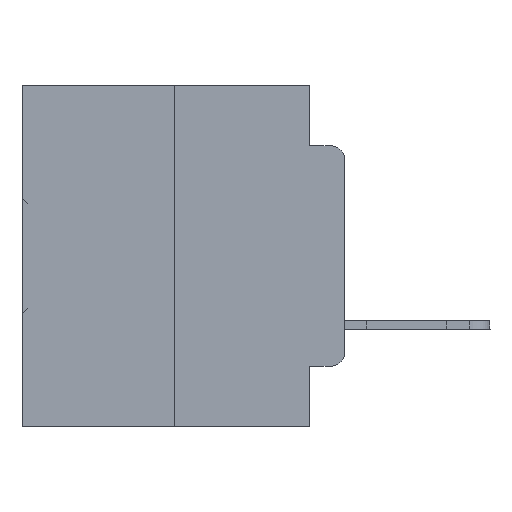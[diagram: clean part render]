
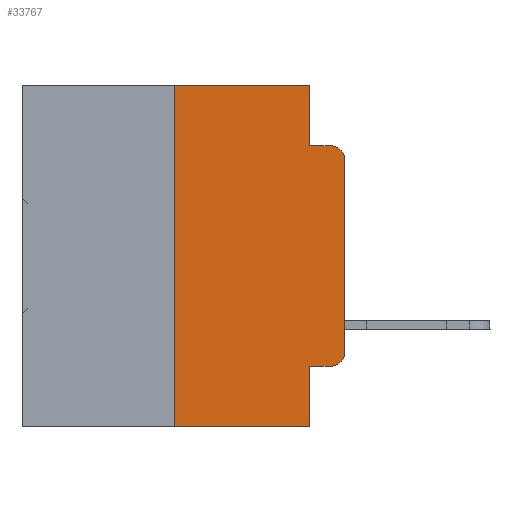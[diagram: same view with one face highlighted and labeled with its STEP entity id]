
A CAD part, left-side view. The second image highlights one B-rep face of the part: STEP entity #33767.
In plain terms, the highlighted planar face has unit normal (-1, 0, 0).
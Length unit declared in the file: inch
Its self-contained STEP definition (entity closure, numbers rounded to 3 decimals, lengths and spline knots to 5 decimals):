
#366 = DIRECTION ( 'NONE',  ( 0., 0., 1. ) ) ;
#1430 = VERTEX_POINT ( 'NONE', #19132 ) ;
#1471 = CARTESIAN_POINT ( 'NONE',  ( 0., 0.051, -0.4115 ) ) ;
#1493 = AXIS2_PLACEMENT_3D ( 'NONE', #34235, #16248, #6735 ) ;
#1638 = EDGE_CURVE ( 'NONE', #22404, #16948, #2850, .T. ) ;
#1696 = LINE ( 'NONE', #15486, #4446 ) ;
#2161 = DIRECTION ( 'NONE',  ( 0., -1., 0. ) ) ;
#2497 = LINE ( 'NONE', #13567, #11631 ) ;
#2709 = CARTESIAN_POINT ( 'NONE',  ( 0., 0.051, 0. ) ) ;
#2835 = ORIENTED_EDGE ( 'NONE', *, *, #12323, .F. ) ;
#2850 = CIRCLE ( 'NONE', #23720, 0.02 ) ;
#3597 = EDGE_CURVE ( 'NONE', #16376, #22404, #8184, .T. ) ;
#3764 = DIRECTION ( 'NONE',  ( 0., 0., 1. ) ) ;
#3869 = EDGE_CURVE ( 'NONE', #33502, #10345, #29828, .T. ) ;
#4326 = VERTEX_POINT ( 'NONE', #13324 ) ;
#4446 = VECTOR ( 'NONE', #26529, 39.37008 ) ;
#4755 = EDGE_CURVE ( 'NONE', #4326, #1430, #1696, .T. ) ;
#5610 = EDGE_CURVE ( 'NONE', #16376, #1430, #15595, .T. ) ;
#5778 = PLANE ( 'NONE',  #19825 ) ;
#5796 = ORIENTED_EDGE ( 'NONE', *, *, #15670, .F. ) ;
#6735 = DIRECTION ( 'NONE',  ( 0., 0., -1. ) ) ;
#7134 = EDGE_LOOP ( 'NONE', ( #18566, #29889, #5796, #25810, #19555, #2835, #34862, #23384, #22696, #13065 ) ) ;
#8184 = LINE ( 'NONE', #18720, #30967 ) ;
#10300 = LINE ( 'NONE', #13361, #29203 ) ;
#10345 = VERTEX_POINT ( 'NONE', #12587 ) ;
#10522 = DIRECTION ( 'NONE',  ( 1., 0., 0. ) ) ;
#11631 = VECTOR ( 'NONE', #2161, 39.37008 ) ;
#12323 = EDGE_CURVE ( 'NONE', #4326, #27994, #22105, .T. ) ;
#12352 = CARTESIAN_POINT ( 'NONE',  ( 0., 0.051, 0. ) ) ;
#12587 = CARTESIAN_POINT ( 'NONE',  ( 0., 0.02, -0.0885 ) ) ;
#13065 = ORIENTED_EDGE ( 'NONE', *, *, #1638, .T. ) ;
#13207 = CARTESIAN_POINT ( 'NONE',  ( 0., 0., -0.3915 ) ) ;
#13252 = CARTESIAN_POINT ( 'NONE',  ( 0., 0.473, 0. ) ) ;
#13324 = CARTESIAN_POINT ( 'NONE',  ( 0., 0.25, -0.5 ) ) ;
#13361 = CARTESIAN_POINT ( 'NONE',  ( 0., 0.051, -0.0885 ) ) ;
#13567 = CARTESIAN_POINT ( 'NONE',  ( 0., 0.473, 0. ) ) ;
#14799 = DIRECTION ( 'NONE',  ( 0., 0., -1. ) ) ;
#15486 = CARTESIAN_POINT ( 'NONE',  ( 0., 0.473, -0.5 ) ) ;
#15595 = LINE ( 'NONE', #26110, #34476 ) ;
#15670 = EDGE_CURVE ( 'NONE', #16125, #10345, #10300, .T. ) ;
#16125 = VERTEX_POINT ( 'NONE', #19430 ) ;
#16248 = DIRECTION ( 'NONE',  ( -1., 0., 0. ) ) ;
#16376 = VERTEX_POINT ( 'NONE', #1471 ) ;
#16539 = VERTEX_POINT ( 'NONE', #2709 ) ;
#16942 = VECTOR ( 'NONE', #17798, 39.37008 ) ;
#16948 = VERTEX_POINT ( 'NONE', #13207 ) ;
#17008 = CARTESIAN_POINT ( 'NONE',  ( 0., 0.02, -0.4115 ) ) ;
#17691 = CARTESIAN_POINT ( 'NONE',  ( 0., 0.02, -0.3915 ) ) ;
#17798 = DIRECTION ( 'NONE',  ( 0., 0., -1. ) ) ;
#18486 = DIRECTION ( 'NONE',  ( 0., 0., -1. ) ) ;
#18566 = ORIENTED_EDGE ( 'NONE', *, *, #35707, .T. ) ;
#18720 = CARTESIAN_POINT ( 'NONE',  ( 0., 0.051, -0.4115 ) ) ;
#19132 = CARTESIAN_POINT ( 'NONE',  ( 0., 0.051, -0.5 ) ) ;
#19430 = CARTESIAN_POINT ( 'NONE',  ( 0., 0.051, -0.0885 ) ) ;
#19555 = ORIENTED_EDGE ( 'NONE', *, *, #31768, .F. ) ;
#19825 = AXIS2_PLACEMENT_3D ( 'NONE', #13252, #10522, #27018 ) ;
#19963 = VECTOR ( 'NONE', #3764, 39.37008 ) ;
#20497 = LINE ( 'NONE', #12352, #16942 ) ;
#22105 = LINE ( 'NONE', #27718, #27798 ) ;
#22404 = VERTEX_POINT ( 'NONE', #17008 ) ;
#22599 = CARTESIAN_POINT ( 'NONE',  ( 0., 0., 0. ) ) ;
#22696 = ORIENTED_EDGE ( 'NONE', *, *, #3597, .T. ) ;
#23384 = ORIENTED_EDGE ( 'NONE', *, *, #5610, .F. ) ;
#23720 = AXIS2_PLACEMENT_3D ( 'NONE', #17691, #34132, #14799 ) ;
#24987 = EDGE_CURVE ( 'NONE', #16539, #16125, #20497, .T. ) ;
#25109 = CARTESIAN_POINT ( 'NONE',  ( 0., 0., -0.1085 ) ) ;
#25117 = CARTESIAN_POINT ( 'NONE',  ( 0., 0.25, 0. ) ) ;
#25810 = ORIENTED_EDGE ( 'NONE', *, *, #24987, .F. ) ;
#26110 = CARTESIAN_POINT ( 'NONE',  ( 0., 0.051, 0. ) ) ;
#26529 = DIRECTION ( 'NONE',  ( 0., -1., 0. ) ) ;
#27018 = DIRECTION ( 'NONE',  ( 0., 0., -1. ) ) ;
#27479 = DIRECTION ( 'NONE',  ( 0., -1., 0. ) ) ;
#27718 = CARTESIAN_POINT ( 'NONE',  ( 0., 0.25, 0. ) ) ;
#27749 = DIRECTION ( 'NONE',  ( 0., -1., 0. ) ) ;
#27798 = VECTOR ( 'NONE', #366, 39.37008 ) ;
#27994 = VERTEX_POINT ( 'NONE', #25117 ) ;
#29203 = VECTOR ( 'NONE', #27479, 39.37008 ) ;
#29828 = CIRCLE ( 'NONE', #1493, 0.02 ) ;
#29889 = ORIENTED_EDGE ( 'NONE', *, *, #3869, .T. ) ;
#30967 = VECTOR ( 'NONE', #27749, 39.37008 ) ;
#31115 = LINE ( 'NONE', #22599, #19963 ) ;
#31768 = EDGE_CURVE ( 'NONE', #27994, #16539, #2497, .T. ) ;
#33502 = VERTEX_POINT ( 'NONE', #25109 ) ;
#33767 = ADVANCED_FACE ( 'NONE', ( #35304 ), #5778, .F. ) ;
#34132 = DIRECTION ( 'NONE',  ( -1., 0., 0. ) ) ;
#34235 = CARTESIAN_POINT ( 'NONE',  ( 0., 0.02, -0.1085 ) ) ;
#34476 = VECTOR ( 'NONE', #18486, 39.37008 ) ;
#34862 = ORIENTED_EDGE ( 'NONE', *, *, #4755, .T. ) ;
#35304 = FACE_OUTER_BOUND ( 'NONE', #7134, .T. ) ;
#35707 = EDGE_CURVE ( 'NONE', #16948, #33502, #31115, .T. ) ;
